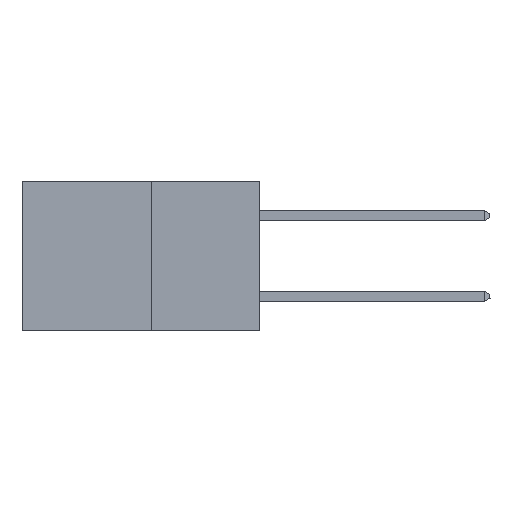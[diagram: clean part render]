
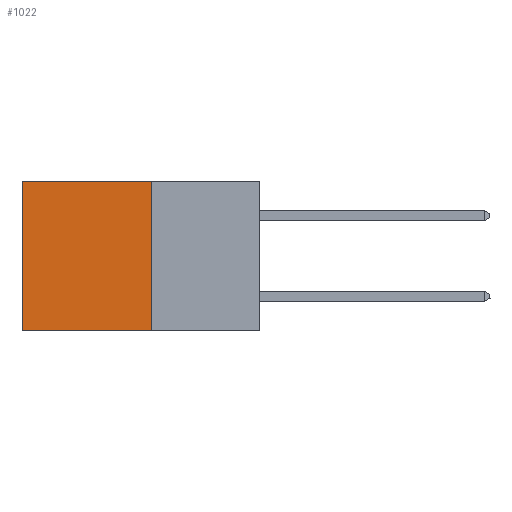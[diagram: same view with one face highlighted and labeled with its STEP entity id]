
A CAD part, left-side view. The second image highlights one B-rep face of the part: STEP entity #1022.
In plain terms, the highlighted planar face has unit normal (-1, 0, 0).
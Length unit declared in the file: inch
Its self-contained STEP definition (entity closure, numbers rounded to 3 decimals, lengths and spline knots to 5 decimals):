
#625 = LINE ( 'NONE', #4289, #18999 ) ;
#1022 = ADVANCED_FACE ( 'NONE', ( #3167 ), #9987, .F. ) ;
#1465 = EDGE_CURVE ( 'NONE', #4580, #7010, #625, .T. ) ;
#1549 = EDGE_CURVE ( 'NONE', #7010, #11519, #20936, .T. ) ;
#2544 = LINE ( 'NONE', #7523, #15756 ) ;
#2555 = ORIENTED_EDGE ( 'NONE', *, *, #1465, .F. ) ;
#2966 = CARTESIAN_POINT ( 'NONE',  ( 0.277, 0.59, -0.37 ) ) ;
#3167 = FACE_OUTER_BOUND ( 'NONE', #21184, .T. ) ;
#3374 = CARTESIAN_POINT ( 'NONE',  ( 0.277, 0.27, -0.37 ) ) ;
#4289 = CARTESIAN_POINT ( 'NONE',  ( 0.277, 0.27, -0.37 ) ) ;
#4580 = VERTEX_POINT ( 'NONE', #18443 ) ;
#7010 = VERTEX_POINT ( 'NONE', #15146 ) ;
#7523 = CARTESIAN_POINT ( 'NONE',  ( 0.277, 0.27, 0. ) ) ;
#7898 = ORIENTED_EDGE ( 'NONE', *, *, #14911, .T. ) ;
#8201 = DIRECTION ( 'NONE',  ( 0., 0., -1. ) ) ;
#8539 = DIRECTION ( 'NONE',  ( 0., 0., -1. ) ) ;
#9211 = DIRECTION ( 'NONE',  ( 0., 1., 0. ) ) ;
#9987 = PLANE ( 'NONE',  #16514 ) ;
#11519 = VERTEX_POINT ( 'NONE', #19653 ) ;
#12640 = EDGE_CURVE ( 'NONE', #4580, #13019, #2544, .T. ) ;
#12787 = VECTOR ( 'NONE', #15730, 39.37008 ) ;
#13003 = DIRECTION ( 'NONE',  ( 0., 0., -1. ) ) ;
#13019 = VERTEX_POINT ( 'NONE', #15033 ) ;
#14142 = ORIENTED_EDGE ( 'NONE', *, *, #12640, .T. ) ;
#14911 = EDGE_CURVE ( 'NONE', #13019, #11519, #16188, .T. ) ;
#15033 = CARTESIAN_POINT ( 'NONE',  ( 0.277, 0.59, 0. ) ) ;
#15146 = CARTESIAN_POINT ( 'NONE',  ( 0.277, 0.27, -0.37 ) ) ;
#15730 = DIRECTION ( 'NONE',  ( 0., 1., 0. ) ) ;
#15756 = VECTOR ( 'NONE', #9211, 39.37008 ) ;
#16188 = LINE ( 'NONE', #2966, #21364 ) ;
#16514 = AXIS2_PLACEMENT_3D ( 'NONE', #21095, #22329, #13003 ) ;
#18172 = ORIENTED_EDGE ( 'NONE', *, *, #1549, .F. ) ;
#18443 = CARTESIAN_POINT ( 'NONE',  ( 0.277, 0.27, 0. ) ) ;
#18999 = VECTOR ( 'NONE', #8539, 39.37008 ) ;
#19653 = CARTESIAN_POINT ( 'NONE',  ( 0.277, 0.59, -0.37 ) ) ;
#20936 = LINE ( 'NONE', #3374, #12787 ) ;
#21095 = CARTESIAN_POINT ( 'NONE',  ( 0.277, 0.27, -0.37 ) ) ;
#21184 = EDGE_LOOP ( 'NONE', ( #7898, #18172, #2555, #14142 ) ) ;
#21364 = VECTOR ( 'NONE', #8201, 39.37008 ) ;
#22329 = DIRECTION ( 'NONE',  ( 1., 0., 0. ) ) ;
